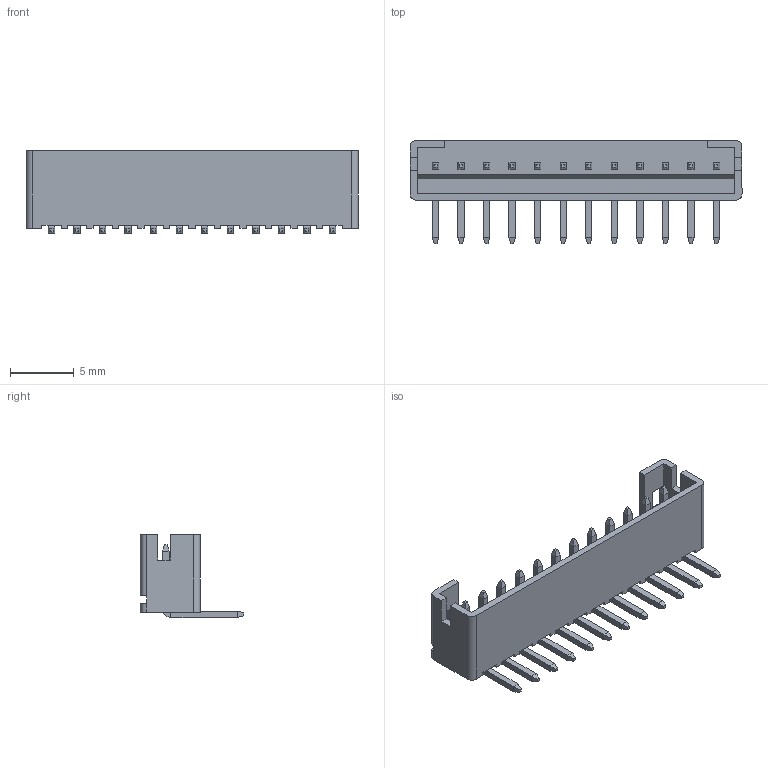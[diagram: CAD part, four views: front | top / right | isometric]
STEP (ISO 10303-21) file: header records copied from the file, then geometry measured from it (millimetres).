
FILE_DESCRIPTION (( 'STEP AP203' ), '1' );
FILE_NAME ('140-512-415-100.STEP', '2020-09-25T11:01:17', ( '' ), ( '' ), 'SwSTEP 2.0', 'SolidWorks 2020', '' );
FILE_SCHEMA (( 'CONFIG_CONTROL_DESIGN' ));
Length unit declared in the file: millimetre
Products named in the file (3): RA LI Housing_512; RA LI Contact_Str; 140-512-415-100
Assembly tree (13 placements, depth 2):
  140-512-415-100
    RA LI Housing_512
    RA LI Contact_Str  x12
Bounding box: 26 x 8.1 x 6.5 mm (x, y, z)
Volume: 278.1 mm3; surface area: 1050.8 mm2
Topology: 13 solids, 13 shells, 400 faces, 932 edges, 556 vertices
Faces by surface type: plane 370, cylinder 30
Entity records: 5721 total; most frequent: CARTESIAN_POINT 914, ORIENTED_EDGE 896, DIRECTION 812, EDGE_CURVE 448, LINE 432, VECTOR 432, VERTEX_POINT 292, AXIS2_PLACEMENT_3D 190
